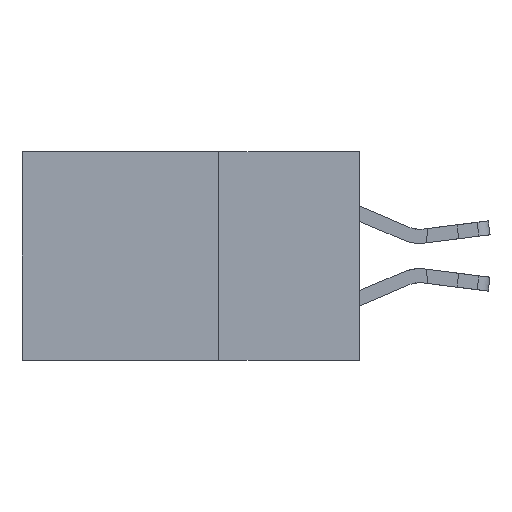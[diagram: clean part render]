
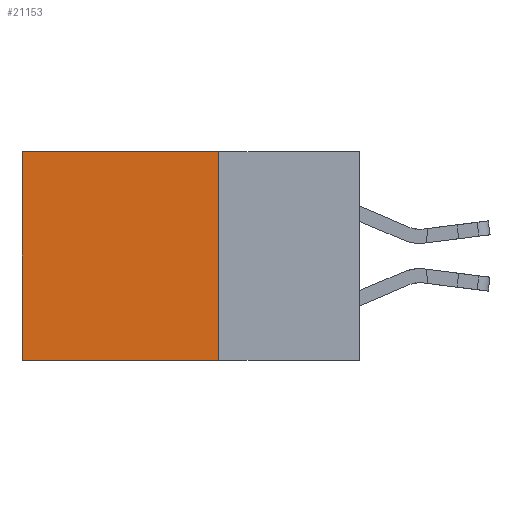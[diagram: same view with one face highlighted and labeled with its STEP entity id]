
A CAD part, left-side view. The second image highlights one B-rep face of the part: STEP entity #21153.
In plain terms, the highlighted planar face has unit normal (-1, 0, 0).
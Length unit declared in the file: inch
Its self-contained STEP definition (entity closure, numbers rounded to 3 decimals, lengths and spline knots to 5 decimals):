
#259 = LINE ( 'NONE', #13519, #11789 ) ;
#412 = CARTESIAN_POINT ( 'NONE',  ( 0.2875, 0.6, 0. ) ) ;
#779 = VERTEX_POINT ( 'NONE', #412 ) ;
#811 = EDGE_CURVE ( 'NONE', #4048, #10185, #9060, .T. ) ;
#3111 = PLANE ( 'NONE',  #3847 ) ;
#3847 = AXIS2_PLACEMENT_3D ( 'NONE', #7311, #20282, #26780 ) ;
#4048 = VERTEX_POINT ( 'NONE', #14944 ) ;
#6158 = EDGE_CURVE ( 'NONE', #18906, #4048, #10641, .T. ) ;
#6810 = ORIENTED_EDGE ( 'NONE', *, *, #25350, .T. ) ;
#7311 = CARTESIAN_POINT ( 'NONE',  ( 0.2875, 0.25, 0. ) ) ;
#8207 = DIRECTION ( 'NONE',  ( 0., 0., -1. ) ) ;
#9060 = LINE ( 'NONE', #17869, #14945 ) ;
#10185 = VERTEX_POINT ( 'NONE', #13468 ) ;
#10231 = EDGE_LOOP ( 'NONE', ( #26577, #11505, #11978, #6810 ) ) ;
#10323 = VECTOR ( 'NONE', #8207, 39.37008 ) ;
#10641 = LINE ( 'NONE', #17146, #10323 ) ;
#11255 = LINE ( 'NONE', #22695, #20626 ) ;
#11505 = ORIENTED_EDGE ( 'NONE', *, *, #811, .F. ) ;
#11789 = VECTOR ( 'NONE', #17868, 39.37008 ) ;
#11978 = ORIENTED_EDGE ( 'NONE', *, *, #6158, .F. ) ;
#12390 = CARTESIAN_POINT ( 'NONE',  ( 0.2875, 0.25, 0. ) ) ;
#13468 = CARTESIAN_POINT ( 'NONE',  ( 0.2875, 0.6, -0.37 ) ) ;
#13519 = CARTESIAN_POINT ( 'NONE',  ( 0.2875, 0.6, 0. ) ) ;
#13569 = DIRECTION ( 'NONE',  ( 0., 1., 0. ) ) ;
#14944 = CARTESIAN_POINT ( 'NONE',  ( 0.2875, 0.25, -0.37 ) ) ;
#14945 = VECTOR ( 'NONE', #26531, 39.37008 ) ;
#17146 = CARTESIAN_POINT ( 'NONE',  ( 0.2875, 0.25, 0. ) ) ;
#17868 = DIRECTION ( 'NONE',  ( 0., 0., -1. ) ) ;
#17869 = CARTESIAN_POINT ( 'NONE',  ( 0.2875, 0.25, -0.37 ) ) ;
#17962 = FACE_OUTER_BOUND ( 'NONE', #10231, .T. ) ;
#18906 = VERTEX_POINT ( 'NONE', #12390 ) ;
#20282 = DIRECTION ( 'NONE',  ( 1., 0., 0. ) ) ;
#20626 = VECTOR ( 'NONE', #13569, 39.37008 ) ;
#21153 = ADVANCED_FACE ( 'NONE', ( #17962 ), #3111, .F. ) ;
#22695 = CARTESIAN_POINT ( 'NONE',  ( 0.2875, 0.25, 0. ) ) ;
#23721 = EDGE_CURVE ( 'NONE', #779, #10185, #259, .T. ) ;
#25350 = EDGE_CURVE ( 'NONE', #18906, #779, #11255, .T. ) ;
#26531 = DIRECTION ( 'NONE',  ( 0., 1., 0. ) ) ;
#26577 = ORIENTED_EDGE ( 'NONE', *, *, #23721, .T. ) ;
#26780 = DIRECTION ( 'NONE',  ( 0., 0., -1. ) ) ;
